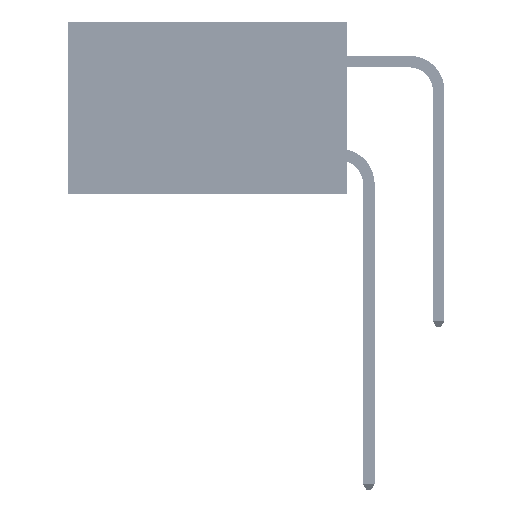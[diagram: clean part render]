
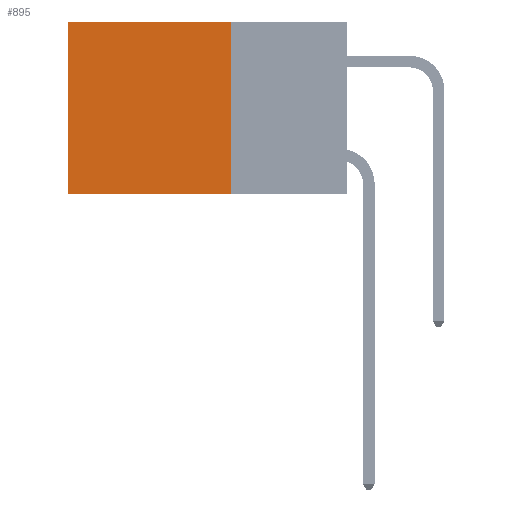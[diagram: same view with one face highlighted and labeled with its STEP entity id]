
A CAD part, left-side view. The second image highlights one B-rep face of the part: STEP entity #895.
In plain terms, the highlighted planar face has unit normal (-1, 0, 0).
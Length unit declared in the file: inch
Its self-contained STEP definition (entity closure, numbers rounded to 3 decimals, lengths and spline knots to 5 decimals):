
#895 = ADVANCED_FACE ( 'NONE', ( #6840 ), #6866, .F. ) ;
#2464 = LINE ( 'NONE', #39494, #26894 ) ;
#5341 = CARTESIAN_POINT ( 'NONE',  ( 0.2875, 0.25, -0.37 ) ) ;
#6840 = FACE_OUTER_BOUND ( 'NONE', #41153, .T. ) ;
#6866 = PLANE ( 'NONE',  #31552 ) ;
#7132 = VECTOR ( 'NONE', #18877, 39.37008 ) ;
#7222 = CARTESIAN_POINT ( 'NONE',  ( 0.2875, 0.25, 0. ) ) ;
#8029 = EDGE_CURVE ( 'NONE', #34839, #48399, #30478, .T. ) ;
#14000 = DIRECTION ( 'NONE',  ( 0., 1., 0. ) ) ;
#15559 = DIRECTION ( 'NONE',  ( 1., 0., 0. ) ) ;
#16147 = VERTEX_POINT ( 'NONE', #34273 ) ;
#16363 = ORIENTED_EDGE ( 'NONE', *, *, #25874, .F. ) ;
#16839 = CARTESIAN_POINT ( 'NONE',  ( 0.2875, 0.6, -0.37 ) ) ;
#18877 = DIRECTION ( 'NONE',  ( 0., 0., -1. ) ) ;
#23409 = EDGE_CURVE ( 'NONE', #16147, #53847, #52081, .T. ) ;
#25874 = EDGE_CURVE ( 'NONE', #48399, #53847, #33751, .T. ) ;
#26894 = VECTOR ( 'NONE', #26926, 39.37008 ) ;
#26926 = DIRECTION ( 'NONE',  ( 0., 1., 0. ) ) ;
#27728 = EDGE_CURVE ( 'NONE', #34839, #16147, #2464, .T. ) ;
#27815 = DIRECTION ( 'NONE',  ( 0., 0., -1. ) ) ;
#30478 = LINE ( 'NONE', #44252, #45666 ) ;
#31552 = AXIS2_PLACEMENT_3D ( 'NONE', #7222, #15559, #48798 ) ;
#33751 = LINE ( 'NONE', #5341, #46913 ) ;
#34273 = CARTESIAN_POINT ( 'NONE',  ( 0.2875, 0.6, 0. ) ) ;
#34839 = VERTEX_POINT ( 'NONE', #43548 ) ;
#35704 = CARTESIAN_POINT ( 'NONE',  ( 0.2875, 0.6, 0. ) ) ;
#36190 = ORIENTED_EDGE ( 'NONE', *, *, #23409, .T. ) ;
#37926 = CARTESIAN_POINT ( 'NONE',  ( 0.2875, 0.25, -0.37 ) ) ;
#39494 = CARTESIAN_POINT ( 'NONE',  ( 0.2875, 0.25, 0. ) ) ;
#41153 = EDGE_LOOP ( 'NONE', ( #36190, #16363, #44553, #42607 ) ) ;
#42607 = ORIENTED_EDGE ( 'NONE', *, *, #27728, .T. ) ;
#43548 = CARTESIAN_POINT ( 'NONE',  ( 0.2875, 0.25, 0. ) ) ;
#44252 = CARTESIAN_POINT ( 'NONE',  ( 0.2875, 0.25, 0. ) ) ;
#44553 = ORIENTED_EDGE ( 'NONE', *, *, #8029, .F. ) ;
#45666 = VECTOR ( 'NONE', #27815, 39.37008 ) ;
#46913 = VECTOR ( 'NONE', #14000, 39.37008 ) ;
#48399 = VERTEX_POINT ( 'NONE', #37926 ) ;
#48798 = DIRECTION ( 'NONE',  ( 0., 0., -1. ) ) ;
#52081 = LINE ( 'NONE', #35704, #7132 ) ;
#53847 = VERTEX_POINT ( 'NONE', #16839 ) ;
